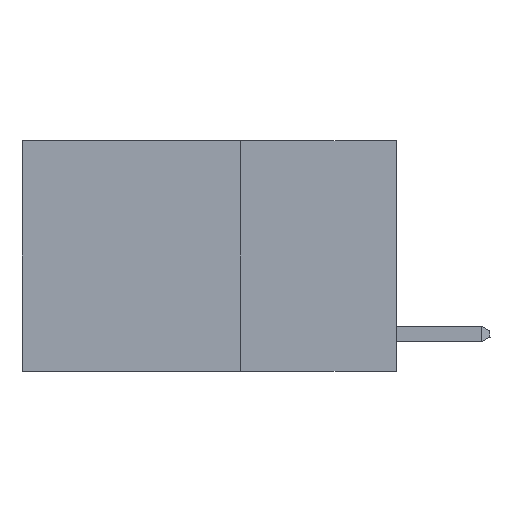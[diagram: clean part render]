
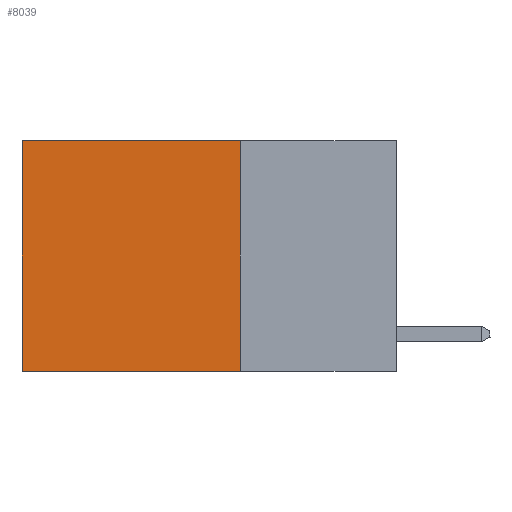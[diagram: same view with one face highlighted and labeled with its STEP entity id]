
A CAD part, left-side view. The second image highlights one B-rep face of the part: STEP entity #8039.
In plain terms, the highlighted planar face has unit normal (-1, 0, 0).
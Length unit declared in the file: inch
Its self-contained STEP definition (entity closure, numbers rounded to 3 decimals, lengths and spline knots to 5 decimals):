
#390 = EDGE_CURVE ( 'NONE', #9264, #26986, #16764, .T. ) ;
#1012 = CARTESIAN_POINT ( 'NONE',  ( 0.2625, 0.25, 0. ) ) ;
#1169 = CARTESIAN_POINT ( 'NONE',  ( 0.2625, 0.25, 0. ) ) ;
#1374 = CARTESIAN_POINT ( 'NONE',  ( 0.2625, 0.25, 0. ) ) ;
#1678 = VERTEX_POINT ( 'NONE', #2452 ) ;
#2452 = CARTESIAN_POINT ( 'NONE',  ( 0.2625, 0.6, 0. ) ) ;
#3446 = DIRECTION ( 'NONE',  ( 0., 1., 0. ) ) ;
#3638 = DIRECTION ( 'NONE',  ( 0., 0., -1. ) ) ;
#3667 = EDGE_CURVE ( 'NONE', #13569, #9264, #22134, .T. ) ;
#4310 = VECTOR ( 'NONE', #16346, 39.37008 ) ;
#6060 = EDGE_LOOP ( 'NONE', ( #16187, #19950, #24432, #10476 ) ) ;
#8039 = ADVANCED_FACE ( 'NONE', ( #14324 ), #14803, .F. ) ;
#9264 = VERTEX_POINT ( 'NONE', #25967 ) ;
#9775 = VECTOR ( 'NONE', #27920, 39.37008 ) ;
#10476 = ORIENTED_EDGE ( 'NONE', *, *, #16899, .T. ) ;
#10853 = VECTOR ( 'NONE', #12202, 39.37008 ) ;
#12202 = DIRECTION ( 'NONE',  ( 0., 1., 0. ) ) ;
#13569 = VERTEX_POINT ( 'NONE', #1012 ) ;
#14324 = FACE_OUTER_BOUND ( 'NONE', #6060, .T. ) ;
#14547 = CARTESIAN_POINT ( 'NONE',  ( 0.2625, 0.6, 0. ) ) ;
#14803 = PLANE ( 'NONE',  #28430 ) ;
#14964 = CARTESIAN_POINT ( 'NONE',  ( 0.2625, 0.6, -0.37 ) ) ;
#15522 = CARTESIAN_POINT ( 'NONE',  ( 0.2625, 0.25, -0.37 ) ) ;
#15672 = LINE ( 'NONE', #14547, #9775 ) ;
#16187 = ORIENTED_EDGE ( 'NONE', *, *, #18181, .T. ) ;
#16346 = DIRECTION ( 'NONE',  ( 0., 0., -1. ) ) ;
#16764 = LINE ( 'NONE', #15522, #10853 ) ;
#16899 = EDGE_CURVE ( 'NONE', #13569, #1678, #23069, .T. ) ;
#17031 = DIRECTION ( 'NONE',  ( 1., 0., 0. ) ) ;
#18181 = EDGE_CURVE ( 'NONE', #1678, #26986, #15672, .T. ) ;
#19950 = ORIENTED_EDGE ( 'NONE', *, *, #390, .F. ) ;
#20971 = VECTOR ( 'NONE', #3446, 39.37008 ) ;
#22134 = LINE ( 'NONE', #27487, #4310 ) ;
#23069 = LINE ( 'NONE', #1169, #20971 ) ;
#24432 = ORIENTED_EDGE ( 'NONE', *, *, #3667, .F. ) ;
#25967 = CARTESIAN_POINT ( 'NONE',  ( 0.2625, 0.25, -0.37 ) ) ;
#26986 = VERTEX_POINT ( 'NONE', #14964 ) ;
#27487 = CARTESIAN_POINT ( 'NONE',  ( 0.2625, 0.25, 0. ) ) ;
#27920 = DIRECTION ( 'NONE',  ( 0., 0., -1. ) ) ;
#28430 = AXIS2_PLACEMENT_3D ( 'NONE', #1374, #17031, #3638 ) ;
